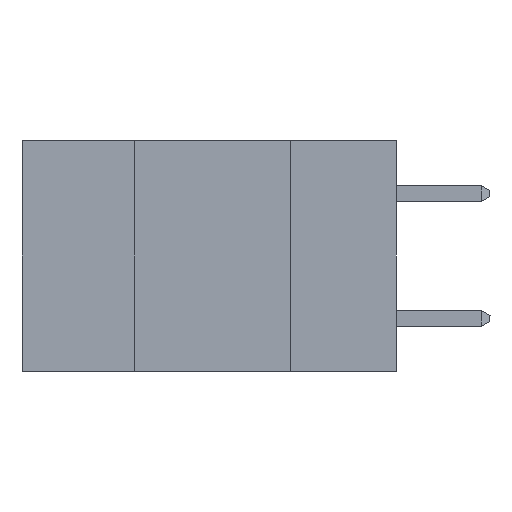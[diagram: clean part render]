
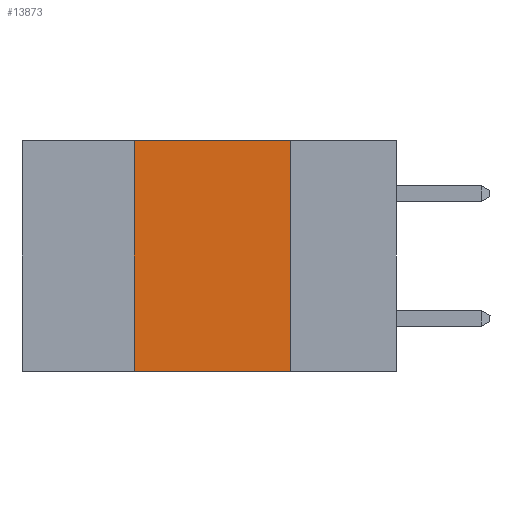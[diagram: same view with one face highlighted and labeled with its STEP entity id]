
A CAD part, left-side view. The second image highlights one B-rep face of the part: STEP entity #13873.
In plain terms, the highlighted planar face has unit normal (-1, 0, 0).
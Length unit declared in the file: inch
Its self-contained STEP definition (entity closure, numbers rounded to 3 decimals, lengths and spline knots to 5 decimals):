
#625 = DIRECTION ( 'NONE',  ( 0., 0., -1. ) ) ;
#996 = LINE ( 'NONE', #13960, #18920 ) ;
#2230 = VERTEX_POINT ( 'NONE', #2719 ) ;
#2331 = ORIENTED_EDGE ( 'NONE', *, *, #5302, .F. ) ;
#2719 = CARTESIAN_POINT ( 'NONE',  ( 0., 0.17, 0. ) ) ;
#4761 = VECTOR ( 'NONE', #20362, 39.37008 ) ;
#5302 = EDGE_CURVE ( 'NONE', #8559, #15213, #996, .T. ) ;
#6211 = VECTOR ( 'NONE', #10114, 39.37008 ) ;
#7989 = EDGE_CURVE ( 'NONE', #15213, #2230, #9823, .T. ) ;
#8559 = VERTEX_POINT ( 'NONE', #18249 ) ;
#8603 = CARTESIAN_POINT ( 'NONE',  ( 0., 0.42, 0. ) ) ;
#8693 = ORIENTED_EDGE ( 'NONE', *, *, #7989, .F. ) ;
#9823 = LINE ( 'NONE', #20526, #4761 ) ;
#9915 = CARTESIAN_POINT ( 'NONE',  ( 0., 0.17, -0.37 ) ) ;
#10114 = DIRECTION ( 'NONE',  ( 0., -1., 0. ) ) ;
#10190 = DIRECTION ( 'NONE',  ( 0., 0., -1. ) ) ;
#10803 = DIRECTION ( 'NONE',  ( 1., 0., 0. ) ) ;
#11211 = VERTEX_POINT ( 'NONE', #9915 ) ;
#11615 = LINE ( 'NONE', #20129, #12147 ) ;
#12147 = VECTOR ( 'NONE', #10190, 39.37008 ) ;
#13873 = ADVANCED_FACE ( 'NONE', ( #18201 ), #15681, .F. ) ;
#13937 = DIRECTION ( 'NONE',  ( 0., 0., 1. ) ) ;
#13960 = CARTESIAN_POINT ( 'NONE',  ( 0., 0.42, -0.37 ) ) ;
#14795 = AXIS2_PLACEMENT_3D ( 'NONE', #20716, #10803, #625 ) ;
#15079 = CARTESIAN_POINT ( 'NONE',  ( 0., 0.6, -0.37 ) ) ;
#15148 = LINE ( 'NONE', #15079, #6211 ) ;
#15213 = VERTEX_POINT ( 'NONE', #8603 ) ;
#15681 = PLANE ( 'NONE',  #14795 ) ;
#16542 = ORIENTED_EDGE ( 'NONE', *, *, #18505, .F. ) ;
#17867 = ORIENTED_EDGE ( 'NONE', *, *, #21375, .T. ) ;
#18201 = FACE_OUTER_BOUND ( 'NONE', #19636, .T. ) ;
#18249 = CARTESIAN_POINT ( 'NONE',  ( 0., 0.42, -0.37 ) ) ;
#18505 = EDGE_CURVE ( 'NONE', #2230, #11211, #11615, .T. ) ;
#18920 = VECTOR ( 'NONE', #13937, 39.37008 ) ;
#19636 = EDGE_LOOP ( 'NONE', ( #16542, #8693, #2331, #17867 ) ) ;
#20129 = CARTESIAN_POINT ( 'NONE',  ( 0., 0.17, -0.37 ) ) ;
#20362 = DIRECTION ( 'NONE',  ( 0., -1., 0. ) ) ;
#20526 = CARTESIAN_POINT ( 'NONE',  ( 0., 0.6, 0. ) ) ;
#20716 = CARTESIAN_POINT ( 'NONE',  ( 0., 0.6, 0. ) ) ;
#21375 = EDGE_CURVE ( 'NONE', #8559, #11211, #15148, .T. ) ;
